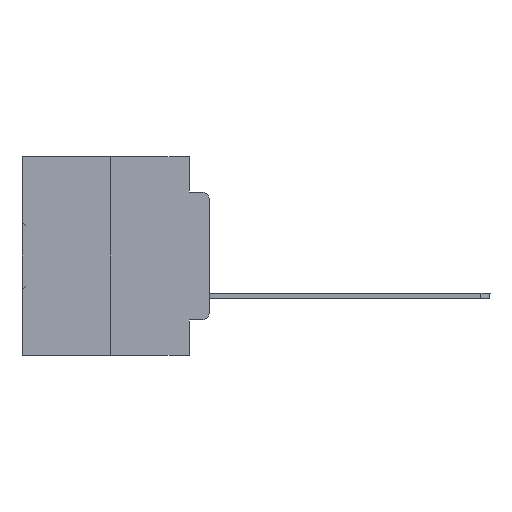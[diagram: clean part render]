
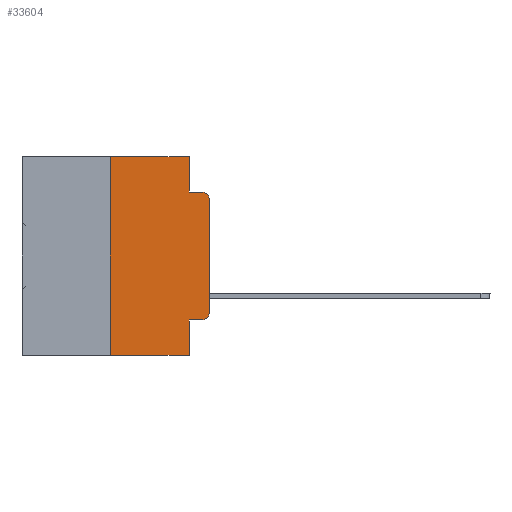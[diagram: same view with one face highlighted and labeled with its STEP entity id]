
A CAD part, left-side view. The second image highlights one B-rep face of the part: STEP entity #33604.
In plain terms, the highlighted planar face has unit normal (-1, 0, 0).
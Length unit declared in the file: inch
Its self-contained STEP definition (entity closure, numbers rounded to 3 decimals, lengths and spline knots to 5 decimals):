
#181 = CARTESIAN_POINT ( 'NONE',  ( 0., 0.051, 0. ) ) ;
#467 = CARTESIAN_POINT ( 'NONE',  ( 0., 0.473, 0. ) ) ;
#691 = LINE ( 'NONE', #23505, #26578 ) ;
#848 = EDGE_CURVE ( 'NONE', #8343, #25175, #30396, .T. ) ;
#1369 = VERTEX_POINT ( 'NONE', #32816 ) ;
#1474 = VECTOR ( 'NONE', #28025, 39.37008 ) ;
#2357 = EDGE_CURVE ( 'NONE', #23797, #30128, #29120, .T. ) ;
#2655 = ORIENTED_EDGE ( 'NONE', *, *, #16350, .T. ) ;
#3336 = ORIENTED_EDGE ( 'NONE', *, *, #26987, .F. ) ;
#3339 = LINE ( 'NONE', #6378, #9911 ) ;
#3506 = CARTESIAN_POINT ( 'NONE',  ( 0., 0., 0. ) ) ;
#3518 = VECTOR ( 'NONE', #31630, 39.37008 ) ;
#4159 = VERTEX_POINT ( 'NONE', #22149 ) ;
#4287 = EDGE_CURVE ( 'NONE', #21344, #10308, #16635, .T. ) ;
#4515 = LINE ( 'NONE', #5787, #1474 ) ;
#5209 = CARTESIAN_POINT ( 'NONE',  ( 0., 0.02, -0.1085 ) ) ;
#5787 = CARTESIAN_POINT ( 'NONE',  ( 0., 0.25, 0. ) ) ;
#6378 = CARTESIAN_POINT ( 'NONE',  ( 0., 0.473, -0.5 ) ) ;
#6526 = ORIENTED_EDGE ( 'NONE', *, *, #35848, .T. ) ;
#7603 = EDGE_CURVE ( 'NONE', #21344, #23797, #691, .T. ) ;
#8207 = AXIS2_PLACEMENT_3D ( 'NONE', #11234, #36157, #22282 ) ;
#8343 = VERTEX_POINT ( 'NONE', #26418 ) ;
#9911 = VECTOR ( 'NONE', #34617, 39.37008 ) ;
#10035 = ORIENTED_EDGE ( 'NONE', *, *, #7603, .T. ) ;
#10308 = VERTEX_POINT ( 'NONE', #31476 ) ;
#10327 = VECTOR ( 'NONE', #23609, 39.37008 ) ;
#10601 = AXIS2_PLACEMENT_3D ( 'NONE', #5209, #30279, #27202 ) ;
#11234 = CARTESIAN_POINT ( 'NONE',  ( 0., 0.473, 0. ) ) ;
#11490 = EDGE_CURVE ( 'NONE', #13228, #1369, #4515, .T. ) ;
#12230 = CARTESIAN_POINT ( 'NONE',  ( 0., 0.02, -0.3915 ) ) ;
#12922 = CARTESIAN_POINT ( 'NONE',  ( 0., 0., -0.3915 ) ) ;
#13228 = VERTEX_POINT ( 'NONE', #25949 ) ;
#13938 = LINE ( 'NONE', #181, #34589 ) ;
#14157 = DIRECTION ( 'NONE',  ( 0., 0., -1. ) ) ;
#14558 = DIRECTION ( 'NONE',  ( 0., -1., 0. ) ) ;
#16074 = ORIENTED_EDGE ( 'NONE', *, *, #2357, .T. ) ;
#16350 = EDGE_CURVE ( 'NONE', #30128, #8343, #27968, .T. ) ;
#16635 = LINE ( 'NONE', #20201, #34648 ) ;
#17109 = CARTESIAN_POINT ( 'NONE',  ( 0., 0.051, -0.0885 ) ) ;
#17204 = AXIS2_PLACEMENT_3D ( 'NONE', #12230, #29063, #17523 ) ;
#17351 = CARTESIAN_POINT ( 'NONE',  ( 0., 0.02, -0.4115 ) ) ;
#17523 = DIRECTION ( 'NONE',  ( 0., 0., -1. ) ) ;
#17712 = DIRECTION ( 'NONE',  ( 0., 0., -1. ) ) ;
#18025 = ORIENTED_EDGE ( 'NONE', *, *, #848, .T. ) ;
#18859 = ORIENTED_EDGE ( 'NONE', *, *, #4287, .F. ) ;
#19468 = PLANE ( 'NONE',  #8207 ) ;
#20201 = CARTESIAN_POINT ( 'NONE',  ( 0., 0.051, 0. ) ) ;
#21344 = VERTEX_POINT ( 'NONE', #24033 ) ;
#22149 = CARTESIAN_POINT ( 'NONE',  ( 0., 0.051, -0.0885 ) ) ;
#22282 = DIRECTION ( 'NONE',  ( 0., 0., -1. ) ) ;
#23144 = DIRECTION ( 'NONE',  ( 0., 0., 1. ) ) ;
#23274 = EDGE_CURVE ( 'NONE', #1369, #26881, #25928, .T. ) ;
#23505 = CARTESIAN_POINT ( 'NONE',  ( 0., 0.051, -0.4115 ) ) ;
#23609 = DIRECTION ( 'NONE',  ( 0., -1., 0. ) ) ;
#23797 = VERTEX_POINT ( 'NONE', #17351 ) ;
#24033 = CARTESIAN_POINT ( 'NONE',  ( 0., 0.051, -0.4115 ) ) ;
#25175 = VERTEX_POINT ( 'NONE', #31882 ) ;
#25928 = LINE ( 'NONE', #467, #3518 ) ;
#25949 = CARTESIAN_POINT ( 'NONE',  ( 0., 0.25, -0.5 ) ) ;
#26418 = CARTESIAN_POINT ( 'NONE',  ( 0., 0., -0.1085 ) ) ;
#26578 = VECTOR ( 'NONE', #14558, 39.37008 ) ;
#26881 = VERTEX_POINT ( 'NONE', #34183 ) ;
#26987 = EDGE_CURVE ( 'NONE', #4159, #25175, #30113, .T. ) ;
#27087 = VECTOR ( 'NONE', #23144, 39.37008 ) ;
#27202 = DIRECTION ( 'NONE',  ( 0., 0., -1. ) ) ;
#27968 = LINE ( 'NONE', #3506, #27087 ) ;
#28025 = DIRECTION ( 'NONE',  ( 0., 0., 1. ) ) ;
#28946 = ORIENTED_EDGE ( 'NONE', *, *, #11490, .F. ) ;
#29063 = DIRECTION ( 'NONE',  ( -1., 0., 0. ) ) ;
#29120 = CIRCLE ( 'NONE', #17204, 0.02 ) ;
#30113 = LINE ( 'NONE', #17109, #10327 ) ;
#30128 = VERTEX_POINT ( 'NONE', #12922 ) ;
#30279 = DIRECTION ( 'NONE',  ( -1., 0., 0. ) ) ;
#30396 = CIRCLE ( 'NONE', #10601, 0.02 ) ;
#31476 = CARTESIAN_POINT ( 'NONE',  ( 0., 0.051, -0.5 ) ) ;
#31630 = DIRECTION ( 'NONE',  ( 0., -1., 0. ) ) ;
#31696 = EDGE_CURVE ( 'NONE', #26881, #4159, #13938, .T. ) ;
#31882 = CARTESIAN_POINT ( 'NONE',  ( 0., 0.02, -0.0885 ) ) ;
#32166 = EDGE_LOOP ( 'NONE', ( #2655, #18025, #3336, #32452, #34374, #28946, #6526, #18859, #10035, #16074 ) ) ;
#32452 = ORIENTED_EDGE ( 'NONE', *, *, #31696, .F. ) ;
#32816 = CARTESIAN_POINT ( 'NONE',  ( 0., 0.25, 0. ) ) ;
#33604 = ADVANCED_FACE ( 'NONE', ( #36012 ), #19468, .F. ) ;
#34183 = CARTESIAN_POINT ( 'NONE',  ( 0., 0.051, 0. ) ) ;
#34374 = ORIENTED_EDGE ( 'NONE', *, *, #23274, .F. ) ;
#34589 = VECTOR ( 'NONE', #14157, 39.37008 ) ;
#34617 = DIRECTION ( 'NONE',  ( 0., -1., 0. ) ) ;
#34648 = VECTOR ( 'NONE', #17712, 39.37008 ) ;
#35848 = EDGE_CURVE ( 'NONE', #13228, #10308, #3339, .T. ) ;
#36012 = FACE_OUTER_BOUND ( 'NONE', #32166, .T. ) ;
#36157 = DIRECTION ( 'NONE',  ( 1., 0., 0. ) ) ;
